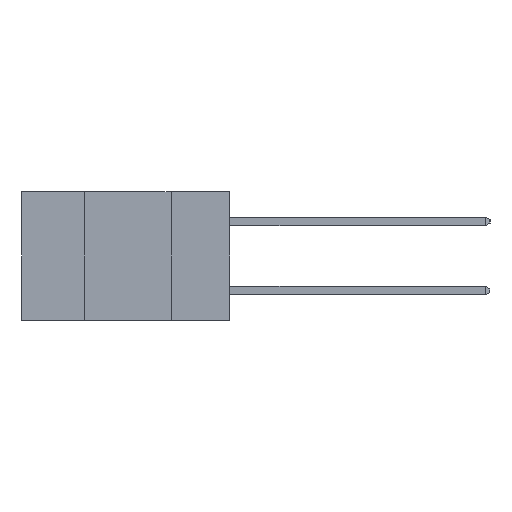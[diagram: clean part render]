
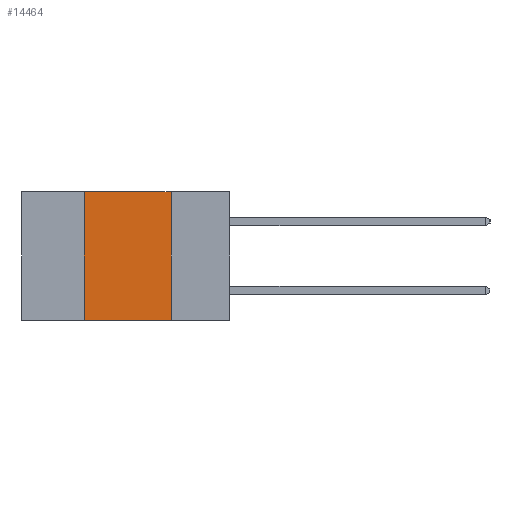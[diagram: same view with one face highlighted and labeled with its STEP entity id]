
A CAD part, left-side view. The second image highlights one B-rep face of the part: STEP entity #14464.
In plain terms, the highlighted planar face has unit normal (-1, 0, 0).
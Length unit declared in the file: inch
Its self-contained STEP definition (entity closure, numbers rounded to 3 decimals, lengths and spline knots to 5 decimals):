
#228 = DIRECTION ( 'NONE',  ( 0., 0., -1. ) ) ;
#1071 = ORIENTED_EDGE ( 'NONE', *, *, #14094, .F. ) ;
#1982 = LINE ( 'NONE', #17164, #5481 ) ;
#2555 = LINE ( 'NONE', #9898, #10082 ) ;
#3179 = CARTESIAN_POINT ( 'NONE',  ( 0., 0.17, -0.37 ) ) ;
#3877 = CARTESIAN_POINT ( 'NONE',  ( 0., 0.42, -0.37 ) ) ;
#4727 = ORIENTED_EDGE ( 'NONE', *, *, #13907, .F. ) ;
#4905 = ORIENTED_EDGE ( 'NONE', *, *, #11335, .F. ) ;
#5150 = ORIENTED_EDGE ( 'NONE', *, *, #10204, .T. ) ;
#5481 = VECTOR ( 'NONE', #7022, 39.37008 ) ;
#6526 = DIRECTION ( 'NONE',  ( 0., -1., 0. ) ) ;
#7022 = DIRECTION ( 'NONE',  ( 0., 0., 1. ) ) ;
#7376 = EDGE_LOOP ( 'NONE', ( #1071, #4727, #4905, #5150 ) ) ;
#7705 = PLANE ( 'NONE',  #8798 ) ;
#8798 = AXIS2_PLACEMENT_3D ( 'NONE', #13536, #9233, #228 ) ;
#9002 = DIRECTION ( 'NONE',  ( 0., -1., 0. ) ) ;
#9151 = VERTEX_POINT ( 'NONE', #18284 ) ;
#9233 = DIRECTION ( 'NONE',  ( 1., 0., 0. ) ) ;
#9898 = CARTESIAN_POINT ( 'NONE',  ( 0., 0.17, 0. ) ) ;
#10082 = VECTOR ( 'NONE', #12783, 39.37008 ) ;
#10204 = EDGE_CURVE ( 'NONE', #15029, #10300, #10798, .T. ) ;
#10300 = VERTEX_POINT ( 'NONE', #3179 ) ;
#10342 = VECTOR ( 'NONE', #9002, 39.37008 ) ;
#10798 = LINE ( 'NONE', #14750, #10342 ) ;
#11335 = EDGE_CURVE ( 'NONE', #15029, #9151, #1982, .T. ) ;
#12783 = DIRECTION ( 'NONE',  ( 0., 0., -1. ) ) ;
#12955 = VERTEX_POINT ( 'NONE', #16063 ) ;
#13229 = LINE ( 'NONE', #15289, #16992 ) ;
#13536 = CARTESIAN_POINT ( 'NONE',  ( 0., 0.6, 0. ) ) ;
#13907 = EDGE_CURVE ( 'NONE', #9151, #12955, #13229, .T. ) ;
#14094 = EDGE_CURVE ( 'NONE', #12955, #10300, #2555, .T. ) ;
#14464 = ADVANCED_FACE ( 'NONE', ( #14783 ), #7705, .F. ) ;
#14750 = CARTESIAN_POINT ( 'NONE',  ( 0., 0.6, -0.37 ) ) ;
#14783 = FACE_OUTER_BOUND ( 'NONE', #7376, .T. ) ;
#15029 = VERTEX_POINT ( 'NONE', #3877 ) ;
#15289 = CARTESIAN_POINT ( 'NONE',  ( 0., 0.6, 0. ) ) ;
#16063 = CARTESIAN_POINT ( 'NONE',  ( 0., 0.17, 0. ) ) ;
#16992 = VECTOR ( 'NONE', #6526, 39.37008 ) ;
#17164 = CARTESIAN_POINT ( 'NONE',  ( 0., 0.42, 0. ) ) ;
#18284 = CARTESIAN_POINT ( 'NONE',  ( 0., 0.42, 0. ) ) ;
